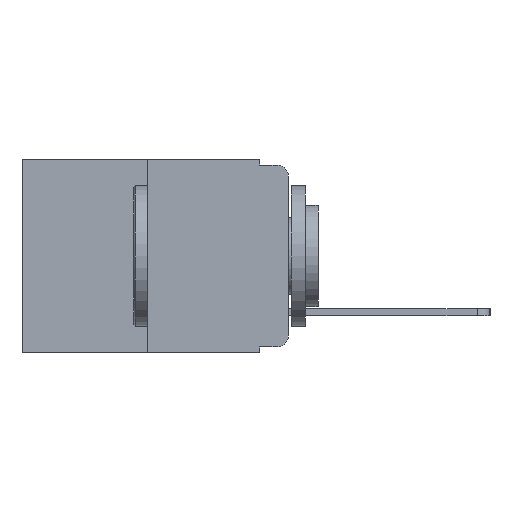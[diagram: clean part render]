
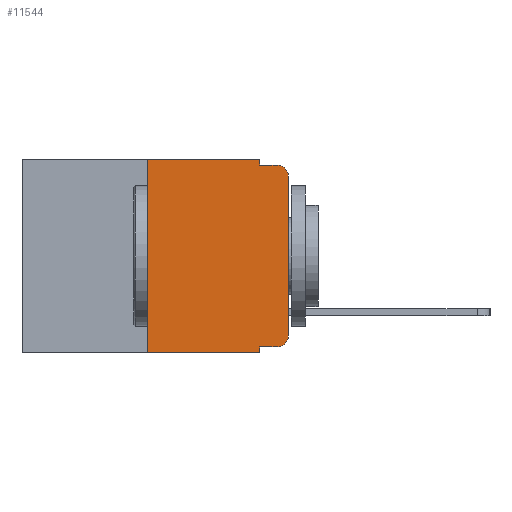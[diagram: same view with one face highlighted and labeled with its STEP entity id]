
A CAD part, left-side view. The second image highlights one B-rep face of the part: STEP entity #11544.
In plain terms, the highlighted planar face has unit normal (-1, 0, 0).
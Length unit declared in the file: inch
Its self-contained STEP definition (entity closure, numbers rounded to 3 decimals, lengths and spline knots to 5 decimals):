
#316 = DIRECTION ( 'NONE',  ( 0., 0., 1. ) ) ;
#376 = VERTEX_POINT ( 'NONE', #16981 ) ;
#684 = CARTESIAN_POINT ( 'NONE',  ( 0., 0.02, -0.03 ) ) ;
#1129 = EDGE_CURVE ( 'NONE', #376, #7357, #24619, .T. ) ;
#1365 = EDGE_CURVE ( 'NONE', #14270, #24475, #20339, .T. ) ;
#1407 = LINE ( 'NONE', #7130, #22625 ) ;
#1521 = AXIS2_PLACEMENT_3D ( 'NONE', #684, #14754, #2763 ) ;
#1968 = CARTESIAN_POINT ( 'NONE',  ( 0., 0.051, 0. ) ) ;
#2253 = LINE ( 'NONE', #3000, #6990 ) ;
#2394 = CARTESIAN_POINT ( 'NONE',  ( 0., 0.25, 0. ) ) ;
#2500 = PLANE ( 'NONE',  #17494 ) ;
#2650 = CARTESIAN_POINT ( 'NONE',  ( 0., 0.051, -0.333 ) ) ;
#2763 = DIRECTION ( 'NONE',  ( 0., 0., -1. ) ) ;
#3000 = CARTESIAN_POINT ( 'NONE',  ( 0., 0.051, -0.01 ) ) ;
#3035 = EDGE_CURVE ( 'NONE', #18186, #12407, #12512, .T. ) ;
#4179 = VECTOR ( 'NONE', #18798, 39.37008 ) ;
#4550 = CARTESIAN_POINT ( 'NONE',  ( 0., 0.473, 0. ) ) ;
#4957 = CARTESIAN_POINT ( 'NONE',  ( 0., 0.051, -0.343 ) ) ;
#5027 = ORIENTED_EDGE ( 'NONE', *, *, #16428, .F. ) ;
#5044 = CARTESIAN_POINT ( 'NONE',  ( 0., 0.051, -0.333 ) ) ;
#5723 = EDGE_CURVE ( 'NONE', #18186, #7294, #15798, .T. ) ;
#6168 = CARTESIAN_POINT ( 'NONE',  ( 0., 0.051, -0.01 ) ) ;
#6572 = DIRECTION ( 'NONE',  ( 0., 0., -1. ) ) ;
#6990 = VECTOR ( 'NONE', #18958, 39.37008 ) ;
#7130 = CARTESIAN_POINT ( 'NONE',  ( 0., 0.473, -0.343 ) ) ;
#7294 = VERTEX_POINT ( 'NONE', #4957 ) ;
#7357 = VERTEX_POINT ( 'NONE', #13154 ) ;
#7508 = ORIENTED_EDGE ( 'NONE', *, *, #1365, .F. ) ;
#7635 = DIRECTION ( 'NONE',  ( 0., -1., 0. ) ) ;
#7681 = VECTOR ( 'NONE', #23818, 39.37008 ) ;
#7712 = LINE ( 'NONE', #2394, #9561 ) ;
#8876 = ORIENTED_EDGE ( 'NONE', *, *, #1129, .T. ) ;
#9561 = VECTOR ( 'NONE', #316, 39.37008 ) ;
#9705 = EDGE_CURVE ( 'NONE', #21158, #14270, #7712, .T. ) ;
#10474 = VECTOR ( 'NONE', #12088, 39.37008 ) ;
#11189 = CARTESIAN_POINT ( 'NONE',  ( 0., 0.02, -0.313 ) ) ;
#11544 = ADVANCED_FACE ( 'NONE', ( #18478 ), #2500, .F. ) ;
#11780 = ORIENTED_EDGE ( 'NONE', *, *, #9705, .F. ) ;
#11988 = EDGE_LOOP ( 'NONE', ( #8876, #19956, #5027, #24494, #7508, #11780, #15015, #20769, #18732, #20067 ) ) ;
#12088 = DIRECTION ( 'NONE',  ( 0., 0., -1. ) ) ;
#12407 = VERTEX_POINT ( 'NONE', #17679 ) ;
#12512 = LINE ( 'NONE', #5044, #22431 ) ;
#12978 = LINE ( 'NONE', #1968, #7681 ) ;
#13154 = CARTESIAN_POINT ( 'NONE',  ( 0., 0., -0.03 ) ) ;
#13211 = DIRECTION ( 'NONE',  ( 0., 0., -1. ) ) ;
#13517 = VERTEX_POINT ( 'NONE', #15112 ) ;
#14143 = VECTOR ( 'NONE', #14252, 39.37008 ) ;
#14252 = DIRECTION ( 'NONE',  ( 0., 0., 1. ) ) ;
#14270 = VERTEX_POINT ( 'NONE', #19401 ) ;
#14492 = VERTEX_POINT ( 'NONE', #6168 ) ;
#14754 = DIRECTION ( 'NONE',  ( -1., 0., 0. ) ) ;
#15015 = ORIENTED_EDGE ( 'NONE', *, *, #21072, .T. ) ;
#15100 = EDGE_CURVE ( 'NONE', #24475, #14492, #12978, .T. ) ;
#15112 = CARTESIAN_POINT ( 'NONE',  ( 0., 0.02, -0.01 ) ) ;
#15798 = LINE ( 'NONE', #23862, #10474 ) ;
#16428 = EDGE_CURVE ( 'NONE', #14492, #13517, #2253, .T. ) ;
#16981 = CARTESIAN_POINT ( 'NONE',  ( 0., 0., -0.313 ) ) ;
#17494 = AXIS2_PLACEMENT_3D ( 'NONE', #4550, #18490, #6572 ) ;
#17679 = CARTESIAN_POINT ( 'NONE',  ( 0., 0.02, -0.333 ) ) ;
#18105 = CARTESIAN_POINT ( 'NONE',  ( 0., 0.473, 0. ) ) ;
#18186 = VERTEX_POINT ( 'NONE', #2650 ) ;
#18478 = FACE_OUTER_BOUND ( 'NONE', #11988, .T. ) ;
#18490 = DIRECTION ( 'NONE',  ( 1., 0., 0. ) ) ;
#18732 = ORIENTED_EDGE ( 'NONE', *, *, #3035, .T. ) ;
#18766 = CARTESIAN_POINT ( 'NONE',  ( 0., 0.051, 0. ) ) ;
#18798 = DIRECTION ( 'NONE',  ( 0., -1., 0. ) ) ;
#18958 = DIRECTION ( 'NONE',  ( 0., -1., 0. ) ) ;
#19401 = CARTESIAN_POINT ( 'NONE',  ( 0., 0.25, 0. ) ) ;
#19628 = CARTESIAN_POINT ( 'NONE',  ( 0., 0., 0. ) ) ;
#19956 = ORIENTED_EDGE ( 'NONE', *, *, #20413, .T. ) ;
#20067 = ORIENTED_EDGE ( 'NONE', *, *, #23505, .T. ) ;
#20339 = LINE ( 'NONE', #18105, #4179 ) ;
#20413 = EDGE_CURVE ( 'NONE', #7357, #13517, #22362, .T. ) ;
#20769 = ORIENTED_EDGE ( 'NONE', *, *, #5723, .F. ) ;
#21042 = DIRECTION ( 'NONE',  ( 0., -1., 0. ) ) ;
#21072 = EDGE_CURVE ( 'NONE', #21158, #7294, #1407, .T. ) ;
#21158 = VERTEX_POINT ( 'NONE', #25193 ) ;
#21473 = AXIS2_PLACEMENT_3D ( 'NONE', #11189, #25006, #13211 ) ;
#22362 = CIRCLE ( 'NONE', #1521, 0.02 ) ;
#22431 = VECTOR ( 'NONE', #7635, 39.37008 ) ;
#22625 = VECTOR ( 'NONE', #21042, 39.37008 ) ;
#23505 = EDGE_CURVE ( 'NONE', #12407, #376, #24055, .T. ) ;
#23818 = DIRECTION ( 'NONE',  ( 0., 0., -1. ) ) ;
#23862 = CARTESIAN_POINT ( 'NONE',  ( 0., 0.051, 0. ) ) ;
#24055 = CIRCLE ( 'NONE', #21473, 0.02 ) ;
#24475 = VERTEX_POINT ( 'NONE', #18766 ) ;
#24494 = ORIENTED_EDGE ( 'NONE', *, *, #15100, .F. ) ;
#24619 = LINE ( 'NONE', #19628, #14143 ) ;
#25006 = DIRECTION ( 'NONE',  ( -1., 0., 0. ) ) ;
#25193 = CARTESIAN_POINT ( 'NONE',  ( 0., 0.25, -0.343 ) ) ;
